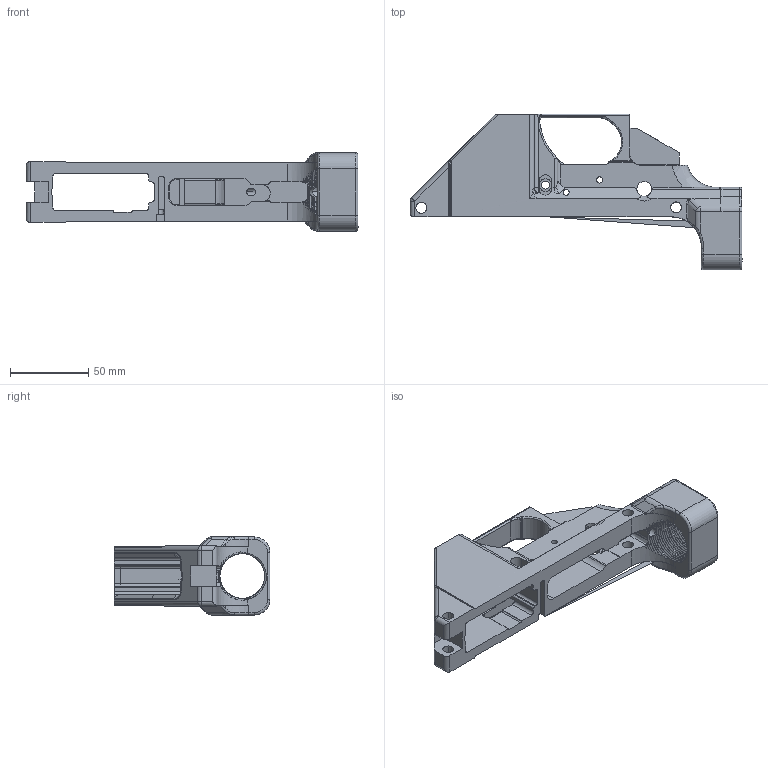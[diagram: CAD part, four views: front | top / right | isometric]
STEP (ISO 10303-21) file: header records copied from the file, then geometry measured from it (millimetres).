
FILE_DESCRIPTION (( 'STEP AP214' ), '1' );
FILE_NAME ('JT_Vanguard_Alter.STEP', '2015-01-03T16:19:12', ( 'WarFairy' ), ( '' ), 'SwSTEP 2.0', 'SolidWorks 2013', '' );
FILE_SCHEMA (( 'AUTOMOTIVE_DESIGN' ));
Length unit declared in the file: millimetre
Products named in the file (1): JT_Vanguard_Alter
Bounding box: 212.37 x 99.72 x 50 mm (x, y, z)
Volume: 178682.1 mm3; surface area: 60662.3 mm2
Topology: 1 solids, 1 shells, 573 faces, 1641 edges, 1051 vertices
Faces by surface type: cylinder 269, plane 144, bspline 133, cone 14, torus 10, sphere 3
Entity records: 46997 total; most frequent: CARTESIAN_POINT 28646, ORIENTED_EDGE 3262, DIRECTION 2183, EDGE_CURVE 1631, VERTEX_POINT 1051, AXIS2_PLACEMENT_3D 791, EDGE_LOOP 602, LINE 601
